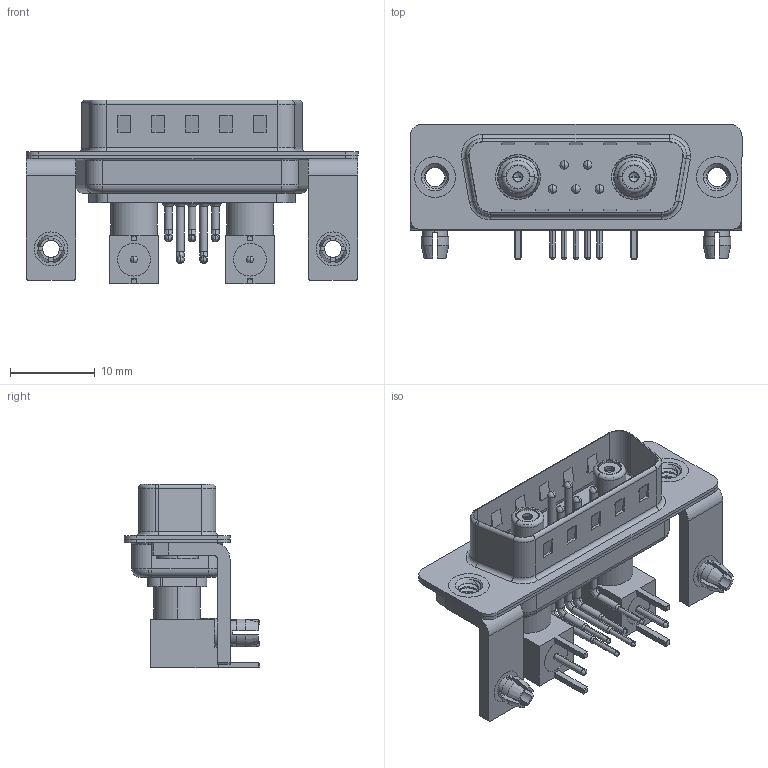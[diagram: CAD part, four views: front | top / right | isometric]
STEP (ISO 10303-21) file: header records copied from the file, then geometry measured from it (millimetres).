
FILE_DESCRIPTION (( 'STEP AP203' ), '1' );
FILE_NAME ('629-7W2-240-7T3.STEP', '2022-05-06T14:20:00', ( '' ), ( '' ), 'SwSTEP 2.0', 'SolidWorks 2020', '' );
FILE_SCHEMA (( 'CONFIG_CONTROL_DESIGN' ));
Length unit declared in the file: millimetre
Products named in the file (18): Co-Ax Jack Assy_RA; Insulator Socket 2; Socket_RA; Co-Ax Jack_RA PC Tail; Locking Collar; Insulator Socket; Insulator RA Pin; 629Combo Contact Row 1; 629Combo Housing_7W2; 629Combo Contact Row 2; 629Combo Shell Front_15 Contacts; 629-7W2-240-7T3; 629Combo Stabilizer Bracket; 629Combo Board Lock; RA Back Shell; 629Combo Threaded Rivet_3; 629Combo Shell Rear_15 Contacts
Assembly tree (30 placements, depth 3):
  629-7W2-240-7T3
    629Combo Housing_7W2
    629Combo Shell Rear_15 Contacts
    629Combo Shell Front_15 Contacts
    629Combo Threaded Rivet_3  x2
    629Combo Stabilizer Bracket  x2
    629Combo Board Lock  x2
    Co-Ax Jack Assy_RA
      Co-Ax Jack_RA PC Tail
      Insulator Socket
      Insulator Socket 2
      Locking Collar
      Socket_RA
      RA Back Shell
      Insulator RA Pin
    Co-Ax Jack Assy_RA
      Co-Ax Jack_RA PC Tail
      Insulator Socket
      Insulator Socket 2
      Locking Collar
      Socket_RA
      RA Back Shell
      Insulator RA Pin
    629Combo Contact Row 1  x2
    629Combo Contact Row 2  x3
Bounding box: 39.2 x 16 x 21.71 mm (x, y, z)
Volume: 2754.6 mm3; surface area: 7580.2 mm2
Topology: 28 solids, 28 shells, 1326 faces, 3451 edges, 2208 vertices
Faces by surface type: plane 641, cylinder 497, cone 84, torus 62, bspline 38, sphere 4
Entity records: 27516 total; most frequent: CARTESIAN_POINT 5923, DIRECTION 4220, ORIENTED_EDGE 3928, EDGE_CURVE 1964, AXIS2_PLACEMENT_3D 1530, VERTEX_POINT 1262, LINE 1160, VECTOR 1160
